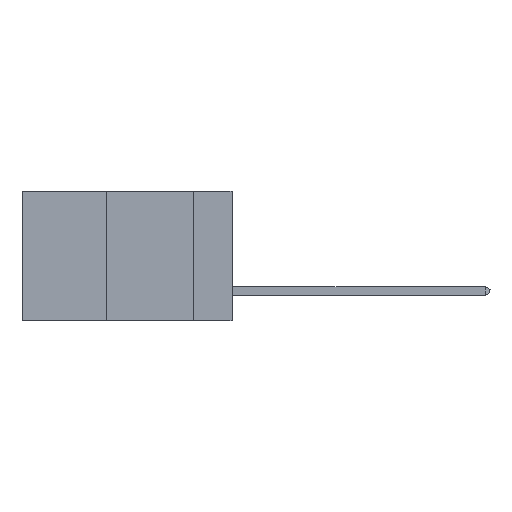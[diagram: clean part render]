
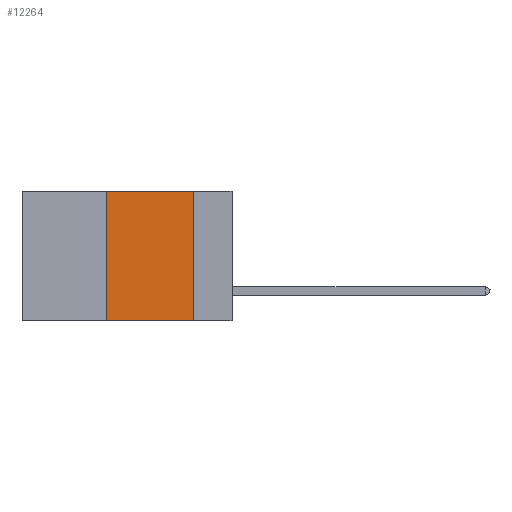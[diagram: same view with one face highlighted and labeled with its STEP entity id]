
A CAD part, left-side view. The second image highlights one B-rep face of the part: STEP entity #12264.
In plain terms, the highlighted planar face has unit normal (-1, 0, 0).
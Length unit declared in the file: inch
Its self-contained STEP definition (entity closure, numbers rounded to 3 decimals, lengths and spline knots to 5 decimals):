
#1961 = VERTEX_POINT ( 'NONE', #32866 ) ;
#2206 = CARTESIAN_POINT ( 'NONE',  ( 0., 0.36, 0. ) ) ;
#2716 = EDGE_CURVE ( 'NONE', #1961, #34187, #5318, .T. ) ;
#2789 = DIRECTION ( 'NONE',  ( 0., -1., 0. ) ) ;
#5318 = LINE ( 'NONE', #10220, #27448 ) ;
#6220 = CARTESIAN_POINT ( 'NONE',  ( 0., 0.36, -0.37 ) ) ;
#7996 = CARTESIAN_POINT ( 'NONE',  ( 0., 0.6, 0. ) ) ;
#10220 = CARTESIAN_POINT ( 'NONE',  ( 0., 0.11, 0. ) ) ;
#10607 = DIRECTION ( 'NONE',  ( 0., 0., -1. ) ) ;
#12201 = VERTEX_POINT ( 'NONE', #15850 ) ;
#12264 = ADVANCED_FACE ( 'NONE', ( #18590 ), #36023, .F. ) ;
#13956 = EDGE_CURVE ( 'NONE', #25089, #12201, #41197, .T. ) ;
#15390 = DIRECTION ( 'NONE',  ( 0., 0., -1. ) ) ;
#15850 = CARTESIAN_POINT ( 'NONE',  ( 0., 0.36, 0. ) ) ;
#18496 = DIRECTION ( 'NONE',  ( 1., 0., 0. ) ) ;
#18590 = FACE_OUTER_BOUND ( 'NONE', #31264, .T. ) ;
#18980 = DIRECTION ( 'NONE',  ( 0., -1., 0. ) ) ;
#20721 = ORIENTED_EDGE ( 'NONE', *, *, #40752, .T. ) ;
#21736 = VECTOR ( 'NONE', #26333, 39.37008 ) ;
#22906 = VECTOR ( 'NONE', #2789, 39.37008 ) ;
#23778 = AXIS2_PLACEMENT_3D ( 'NONE', #7996, #18496, #15390 ) ;
#25089 = VERTEX_POINT ( 'NONE', #6220 ) ;
#26333 = DIRECTION ( 'NONE',  ( 0., 0., 1. ) ) ;
#27448 = VECTOR ( 'NONE', #10607, 39.37008 ) ;
#30075 = LINE ( 'NONE', #36195, #38143 ) ;
#31264 = EDGE_LOOP ( 'NONE', ( #32391, #40921, #38786, #20721 ) ) ;
#32391 = ORIENTED_EDGE ( 'NONE', *, *, #2716, .F. ) ;
#32866 = CARTESIAN_POINT ( 'NONE',  ( 0., 0.11, 0. ) ) ;
#34051 = EDGE_CURVE ( 'NONE', #12201, #1961, #30075, .T. ) ;
#34187 = VERTEX_POINT ( 'NONE', #38462 ) ;
#36023 = PLANE ( 'NONE',  #23778 ) ;
#36195 = CARTESIAN_POINT ( 'NONE',  ( 0., 0.6, 0. ) ) ;
#38143 = VECTOR ( 'NONE', #18980, 39.37008 ) ;
#38462 = CARTESIAN_POINT ( 'NONE',  ( 0., 0.11, -0.37 ) ) ;
#38786 = ORIENTED_EDGE ( 'NONE', *, *, #13956, .F. ) ;
#40752 = EDGE_CURVE ( 'NONE', #25089, #34187, #43345, .T. ) ;
#40921 = ORIENTED_EDGE ( 'NONE', *, *, #34051, .F. ) ;
#41181 = CARTESIAN_POINT ( 'NONE',  ( 0., 0.6, -0.37 ) ) ;
#41197 = LINE ( 'NONE', #2206, #21736 ) ;
#43345 = LINE ( 'NONE', #41181, #22906 ) ;
